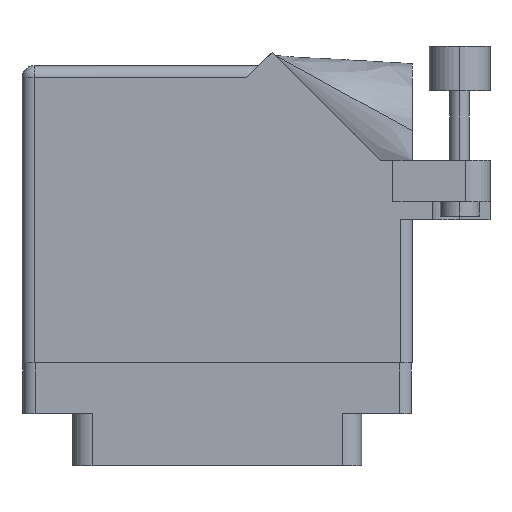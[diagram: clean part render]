
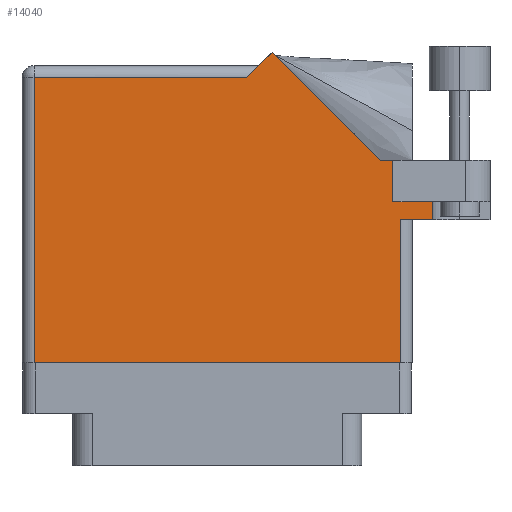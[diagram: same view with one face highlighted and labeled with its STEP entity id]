
A CAD part, front view. The second image highlights one B-rep face of the part: STEP entity #14040.
In plain terms, the highlighted face is planar.
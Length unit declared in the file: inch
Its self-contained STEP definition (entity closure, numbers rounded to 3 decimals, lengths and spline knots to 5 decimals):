
#1151 = DIRECTION ( 'NONE',  ( 1., 0., 0. ) ) ;
#1282 = CARTESIAN_POINT ( 'NONE',  ( 1.84442, 1.044, 0. ) ) ;
#1671 = FACE_OUTER_BOUND ( 'NONE', #8852, .T. ) ;
#2010 = CARTESIAN_POINT ( 'NONE',  ( 1.84442, 1.044, 0. ) ) ;
#2419 = AXIS2_PLACEMENT_3D ( 'NONE', #22210, #25498, #34171 ) ;
#2451 = VECTOR ( 'NONE', #24631, 39.37008 ) ;
#2831 = ORIENTED_EDGE ( 'NONE', *, *, #10145, .T. ) ;
#3047 = CARTESIAN_POINT ( 'NONE',  ( 0., 1.468, 0. ) ) ;
#3413 = EDGE_CURVE ( 'NONE', #10690, #25325, #39296, .T. ) ;
#3800 = CARTESIAN_POINT ( 'NONE',  ( 1.28771, 1.60071, 0. ) ) ;
#4120 = EDGE_CURVE ( 'NONE', #24143, #8149, #15457, .T. ) ;
#4355 = CARTESIAN_POINT ( 'NONE',  ( 0., 0., 0. ) ) ;
#4665 = LINE ( 'NONE', #39128, #32184 ) ;
#4780 = EDGE_CURVE ( 'NONE', #13715, #8149, #9725, .T. ) ;
#6529 = CARTESIAN_POINT ( 'NONE',  ( 2.1115, 1.16177, 0. ) ) ;
#6591 = DIRECTION ( 'NONE',  ( 0., 1., 0. ) ) ;
#7079 = VECTOR ( 'NONE', #8194, 39.37008 ) ;
#7282 = ORIENTED_EDGE ( 'NONE', *, *, #3413, .T. ) ;
#7942 = CARTESIAN_POINT ( 'NONE',  ( 1.155, 1.468, 0. ) ) ;
#8149 = VERTEX_POINT ( 'NONE', #26977 ) ;
#8194 = DIRECTION ( 'NONE',  ( 0., 1., 0. ) ) ;
#8268 = VECTOR ( 'NONE', #1151, 39.37008 ) ;
#8732 = ORIENTED_EDGE ( 'NONE', *, *, #33210, .T. ) ;
#8852 = EDGE_LOOP ( 'NONE', ( #17024, #28675, #29594, #35838, #35443, #8732, #7282, #22223, #2831, #27391, #11656 ) ) ;
#8937 = CARTESIAN_POINT ( 'NONE',  ( 0.062, 0., 0. ) ) ;
#9725 = LINE ( 'NONE', #37536, #8268 ) ;
#9749 = DIRECTION ( 'NONE',  ( -0.707, -0.707, 0. ) ) ;
#9849 = DIRECTION ( 'NONE',  ( 0., -1., 0. ) ) ;
#10145 = EDGE_CURVE ( 'NONE', #33958, #14459, #32450, .T. ) ;
#10690 = VERTEX_POINT ( 'NONE', #20449 ) ;
#11656 = ORIENTED_EDGE ( 'NONE', *, *, #33914, .T. ) ;
#12366 = EDGE_CURVE ( 'NONE', #20280, #24143, #20317, .T. ) ;
#13213 = DIRECTION ( 'NONE',  ( 1., 0., 0. ) ) ;
#13715 = VERTEX_POINT ( 'NONE', #36901 ) ;
#14040 = ADVANCED_FACE ( 'NONE', ( #1671 ), #31371, .F. ) ;
#14459 = VERTEX_POINT ( 'NONE', #7942 ) ;
#15052 = EDGE_CURVE ( 'NONE', #29378, #20279, #23422, .T. ) ;
#15457 = LINE ( 'NONE', #6529, #38310 ) ;
#17024 = ORIENTED_EDGE ( 'NONE', *, *, #15052, .T. ) ;
#18207 = DIRECTION ( 'NONE',  ( 0., -1., 0. ) ) ;
#18348 = EDGE_CURVE ( 'NONE', #25325, #33958, #35135, .T. ) ;
#18621 = CARTESIAN_POINT ( 'NONE',  ( 1.217, 1.53, 0. ) ) ;
#20279 = VERTEX_POINT ( 'NONE', #31373 ) ;
#20280 = VERTEX_POINT ( 'NONE', #31234 ) ;
#20317 = LINE ( 'NONE', #38326, #21764 ) ;
#20449 = CARTESIAN_POINT ( 'NONE',  ( 1.91, 1.044, 0. ) ) ;
#21764 = VECTOR ( 'NONE', #31661, 39.37008 ) ;
#21892 = LINE ( 'NONE', #3047, #2451 ) ;
#22210 = CARTESIAN_POINT ( 'NONE',  ( 0., 1.53, 0. ) ) ;
#22223 = ORIENTED_EDGE ( 'NONE', *, *, #18348, .T. ) ;
#23422 = LINE ( 'NONE', #4355, #25771 ) ;
#23881 = VECTOR ( 'NONE', #9749, 39.37008 ) ;
#24143 = VERTEX_POINT ( 'NONE', #37354 ) ;
#24631 = DIRECTION ( 'NONE',  ( -1., 0., 0. ) ) ;
#25325 = VERTEX_POINT ( 'NONE', #1282 ) ;
#25385 = CARTESIAN_POINT ( 'NONE',  ( 0.062, 1.468, 0. ) ) ;
#25419 = VERTEX_POINT ( 'NONE', #25385 ) ;
#25498 = DIRECTION ( 'NONE',  ( 0., 0., -1. ) ) ;
#25771 = VECTOR ( 'NONE', #13213, 39.37008 ) ;
#26064 = LINE ( 'NONE', #38630, #7079 ) ;
#26381 = CARTESIAN_POINT ( 'NONE',  ( 0.062, 0., 0. ) ) ;
#26939 = VECTOR ( 'NONE', #33893, 39.37008 ) ;
#26977 = CARTESIAN_POINT ( 'NONE',  ( 2.1115, 0.737, 0. ) ) ;
#27391 = ORIENTED_EDGE ( 'NONE', *, *, #31413, .T. ) ;
#27483 = EDGE_CURVE ( 'NONE', #20279, #13715, #4665, .T. ) ;
#27749 = CARTESIAN_POINT ( 'NONE',  ( 2.41, 1.044, 0. ) ) ;
#28387 = VECTOR ( 'NONE', #18207, 39.37008 ) ;
#28675 = ORIENTED_EDGE ( 'NONE', *, *, #27483, .T. ) ;
#29378 = VERTEX_POINT ( 'NONE', #26381 ) ;
#29594 = ORIENTED_EDGE ( 'NONE', *, *, #4780, .T. ) ;
#31234 = CARTESIAN_POINT ( 'NONE',  ( 1.91, 0.831, 0. ) ) ;
#31371 = PLANE ( 'NONE',  #2419 ) ;
#31373 = CARTESIAN_POINT ( 'NONE',  ( 1.948, 0., 0. ) ) ;
#31413 = EDGE_CURVE ( 'NONE', #14459, #25419, #21892, .T. ) ;
#31661 = DIRECTION ( 'NONE',  ( 1., 0., 0. ) ) ;
#32184 = VECTOR ( 'NONE', #6591, 39.37008 ) ;
#32267 = VECTOR ( 'NONE', #38390, 39.37008 ) ;
#32450 = LINE ( 'NONE', #18621, #23881 ) ;
#33210 = EDGE_CURVE ( 'NONE', #20280, #10690, #26064, .T. ) ;
#33893 = DIRECTION ( 'NONE',  ( -1., 0., 0. ) ) ;
#33914 = EDGE_CURVE ( 'NONE', #25419, #29378, #37940, .T. ) ;
#33958 = VERTEX_POINT ( 'NONE', #3800 ) ;
#34171 = DIRECTION ( 'NONE',  ( -1., 0., 0. ) ) ;
#35135 = LINE ( 'NONE', #2010, #32267 ) ;
#35443 = ORIENTED_EDGE ( 'NONE', *, *, #12366, .F. ) ;
#35838 = ORIENTED_EDGE ( 'NONE', *, *, #4120, .F. ) ;
#36901 = CARTESIAN_POINT ( 'NONE',  ( 1.948, 0.737, 0. ) ) ;
#37354 = CARTESIAN_POINT ( 'NONE',  ( 2.1115, 0.831, 0. ) ) ;
#37536 = CARTESIAN_POINT ( 'NONE',  ( 2.01, 0.737, 0. ) ) ;
#37940 = LINE ( 'NONE', #8937, #28387 ) ;
#38310 = VECTOR ( 'NONE', #9849, 39.37008 ) ;
#38326 = CARTESIAN_POINT ( 'NONE',  ( 1.91, 0.831, 0. ) ) ;
#38390 = DIRECTION ( 'NONE',  ( -0.707, 0.707, 0. ) ) ;
#38630 = CARTESIAN_POINT ( 'NONE',  ( 1.91, 0.831, 0. ) ) ;
#39128 = CARTESIAN_POINT ( 'NONE',  ( 1.948, 0.737, 0. ) ) ;
#39296 = LINE ( 'NONE', #27749, #26939 ) ;
